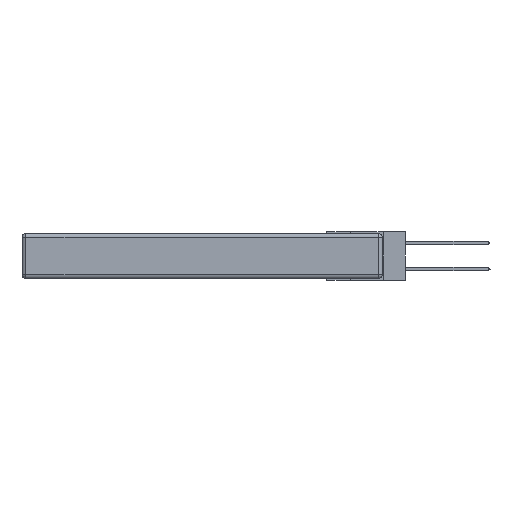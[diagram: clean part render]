
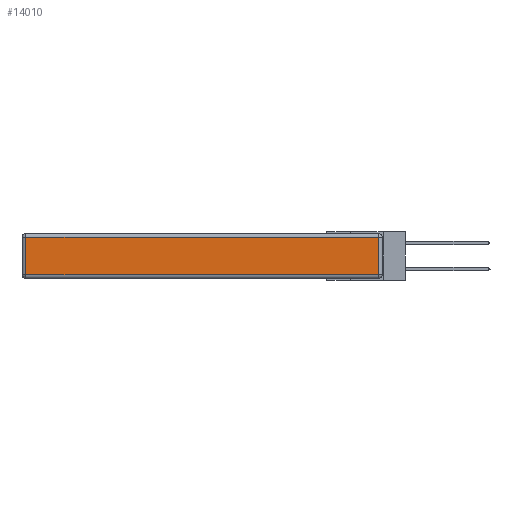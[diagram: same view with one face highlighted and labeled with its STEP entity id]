
A CAD part, left-side view. The second image highlights one B-rep face of the part: STEP entity #14010.
In plain terms, the highlighted planar face has unit normal (-1, 0, 0).
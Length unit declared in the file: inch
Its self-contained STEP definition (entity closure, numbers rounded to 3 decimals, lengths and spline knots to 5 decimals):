
#621 = ORIENTED_EDGE ( 'NONE', *, *, #8869, .T. ) ;
#688 = LINE ( 'NONE', #3236, #16571 ) ;
#981 = EDGE_LOOP ( 'NONE', ( #621, #4753, #12583, #19135 ) ) ;
#2792 = VECTOR ( 'NONE', #14050, 39.37008 ) ;
#3236 = CARTESIAN_POINT ( 'NONE',  ( 0., 2.72, -0.343 ) ) ;
#3425 = CARTESIAN_POINT ( 'NONE',  ( 0., 0., -0.313 ) ) ;
#3963 = CARTESIAN_POINT ( 'NONE',  ( 0., 0.03, -0.03 ) ) ;
#4108 = LINE ( 'NONE', #13621, #15546 ) ;
#4753 = ORIENTED_EDGE ( 'NONE', *, *, #10932, .T. ) ;
#5381 = LINE ( 'NONE', #11073, #2792 ) ;
#5530 = EDGE_CURVE ( 'NONE', #6788, #10244, #4108, .T. ) ;
#6788 = VERTEX_POINT ( 'NONE', #3963 ) ;
#7135 = VECTOR ( 'NONE', #9639, 39.37008 ) ;
#7548 = DIRECTION ( 'NONE',  ( 0., 0., 1. ) ) ;
#7738 = VERTEX_POINT ( 'NONE', #8681 ) ;
#8681 = CARTESIAN_POINT ( 'NONE',  ( 0., 2.72, -0.313 ) ) ;
#8869 = EDGE_CURVE ( 'NONE', #7738, #13857, #12254, .T. ) ;
#8996 = DIRECTION ( 'NONE',  ( 0., 0., -1. ) ) ;
#9568 = AXIS2_PLACEMENT_3D ( 'NONE', #11758, #10271, #7548 ) ;
#9639 = DIRECTION ( 'NONE',  ( 0., -1., 0. ) ) ;
#10244 = VERTEX_POINT ( 'NONE', #13119 ) ;
#10271 = DIRECTION ( 'NONE',  ( -1., 0., 0. ) ) ;
#10932 = EDGE_CURVE ( 'NONE', #13857, #6788, #5381, .T. ) ;
#11073 = CARTESIAN_POINT ( 'NONE',  ( 0., 0.03, -0.343 ) ) ;
#11758 = CARTESIAN_POINT ( 'NONE',  ( 0., 0., -0.343 ) ) ;
#12254 = LINE ( 'NONE', #3425, #7135 ) ;
#12583 = ORIENTED_EDGE ( 'NONE', *, *, #5530, .T. ) ;
#12971 = CARTESIAN_POINT ( 'NONE',  ( 0., 0.03, -0.313 ) ) ;
#13119 = CARTESIAN_POINT ( 'NONE',  ( 0., 2.72, -0.03 ) ) ;
#13621 = CARTESIAN_POINT ( 'NONE',  ( 0., 2.75, -0.03 ) ) ;
#13857 = VERTEX_POINT ( 'NONE', #12971 ) ;
#14010 = ADVANCED_FACE ( 'NONE', ( #17810 ), #16255, .T. ) ;
#14050 = DIRECTION ( 'NONE',  ( 0., 0., 1. ) ) ;
#15225 = DIRECTION ( 'NONE',  ( 0., 1., 0. ) ) ;
#15475 = EDGE_CURVE ( 'NONE', #10244, #7738, #688, .T. ) ;
#15546 = VECTOR ( 'NONE', #15225, 39.37008 ) ;
#16255 = PLANE ( 'NONE',  #9568 ) ;
#16571 = VECTOR ( 'NONE', #8996, 39.37008 ) ;
#17810 = FACE_OUTER_BOUND ( 'NONE', #981, .T. ) ;
#19135 = ORIENTED_EDGE ( 'NONE', *, *, #15475, .T. ) ;
